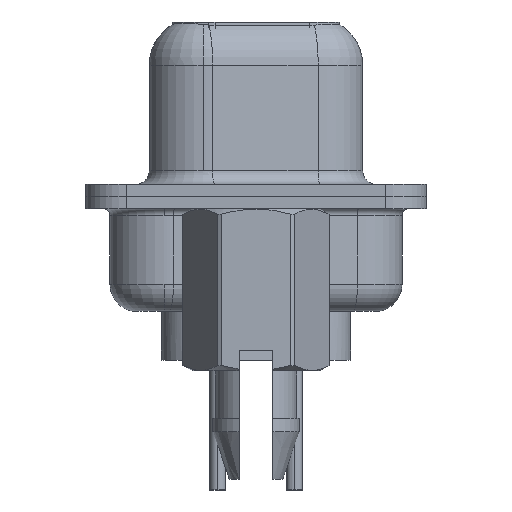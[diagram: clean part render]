
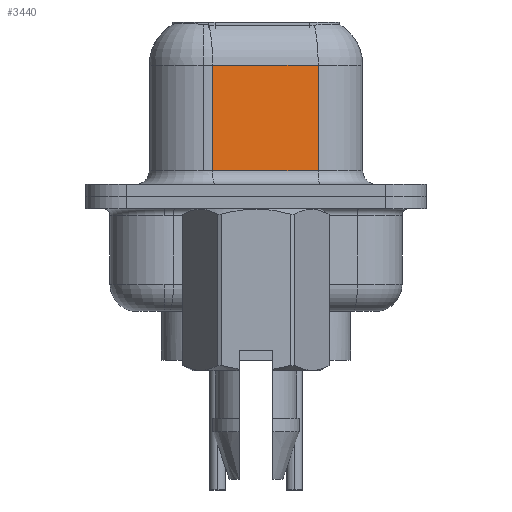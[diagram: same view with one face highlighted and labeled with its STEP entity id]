
A CAD part, left-side view. The second image highlights one B-rep face of the part: STEP entity #3440.
In plain terms, the highlighted planar face has unit normal (-0.985, -0.174, 0).
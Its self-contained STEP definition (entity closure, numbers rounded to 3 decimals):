
#552 = CARTESIAN_POINT ( 'NONE',  ( 4.365, 1.603, 0.95 ) ) ;
#1580 = CARTESIAN_POINT ( 'NONE',  ( 5.053, -2.297, 6.6 ) ) ;
#1844 = DIRECTION ( 'NONE',  ( 0., 0., -1. ) ) ;
#2381 = CARTESIAN_POINT ( 'NONE',  ( 5.053, -2.297, 0.95 ) ) ;
#3440 = ADVANCED_FACE ( 'NONE', ( #22589 ), #24503, .F. ) ;
#3803 = VECTOR ( 'NONE', #12939, 1000. ) ;
#4145 = EDGE_CURVE ( 'NONE', #16629, #17598, #10464, .T. ) ;
#6991 = AXIS2_PLACEMENT_3D ( 'NONE', #11397, #20933, #7047 ) ;
#7047 = DIRECTION ( 'NONE',  ( -0.174, 0.985, 0. ) ) ;
#7150 = EDGE_CURVE ( 'NONE', #21268, #20339, #16501, .T. ) ;
#8665 = EDGE_LOOP ( 'NONE', ( #9458, #25074, #15502, #9904 ) ) ;
#9458 = ORIENTED_EDGE ( 'NONE', *, *, #21196, .F. ) ;
#9904 = ORIENTED_EDGE ( 'NONE', *, *, #7150, .T. ) ;
#10464 = LINE ( 'NONE', #10589, #16406 ) ;
#10467 = VECTOR ( 'NONE', #1844, 1000. ) ;
#10589 = CARTESIAN_POINT ( 'NONE',  ( 5.053, -2.297, 4.85 ) ) ;
#11397 = CARTESIAN_POINT ( 'NONE',  ( 5.053, -2.297, 6.6 ) ) ;
#12939 = DIRECTION ( 'NONE',  ( 0.174, -0.985, 0. ) ) ;
#13139 = CARTESIAN_POINT ( 'NONE',  ( 4.365, 1.603, 6.6 ) ) ;
#15502 = ORIENTED_EDGE ( 'NONE', *, *, #21087, .T. ) ;
#15754 = VECTOR ( 'NONE', #17194, 1000. ) ;
#16406 = VECTOR ( 'NONE', #18683, 1000. ) ;
#16501 = LINE ( 'NONE', #24490, #3803 ) ;
#16629 = VERTEX_POINT ( 'NONE', #25021 ) ;
#17194 = DIRECTION ( 'NONE',  ( 0., 0., -1. ) ) ;
#17321 = LINE ( 'NONE', #13139, #10467 ) ;
#17447 = CARTESIAN_POINT ( 'NONE',  ( 4.365, 1.603, 4.85 ) ) ;
#17598 = VERTEX_POINT ( 'NONE', #17447 ) ;
#18683 = DIRECTION ( 'NONE',  ( -0.174, 0.985, 0. ) ) ;
#19092 = LINE ( 'NONE', #1580, #15754 ) ;
#20339 = VERTEX_POINT ( 'NONE', #2381 ) ;
#20933 = DIRECTION ( 'NONE',  ( 0.985, 0.174, 0. ) ) ;
#21087 = EDGE_CURVE ( 'NONE', #17598, #21268, #17321, .T. ) ;
#21196 = EDGE_CURVE ( 'NONE', #16629, #20339, #19092, .T. ) ;
#21268 = VERTEX_POINT ( 'NONE', #552 ) ;
#22589 = FACE_OUTER_BOUND ( 'NONE', #8665, .T. ) ;
#24490 = CARTESIAN_POINT ( 'NONE',  ( 5.053, -2.297, 0.95 ) ) ;
#24503 = PLANE ( 'NONE',  #6991 ) ;
#25021 = CARTESIAN_POINT ( 'NONE',  ( 5.053, -2.297, 4.85 ) ) ;
#25074 = ORIENTED_EDGE ( 'NONE', *, *, #4145, .T. ) ;
